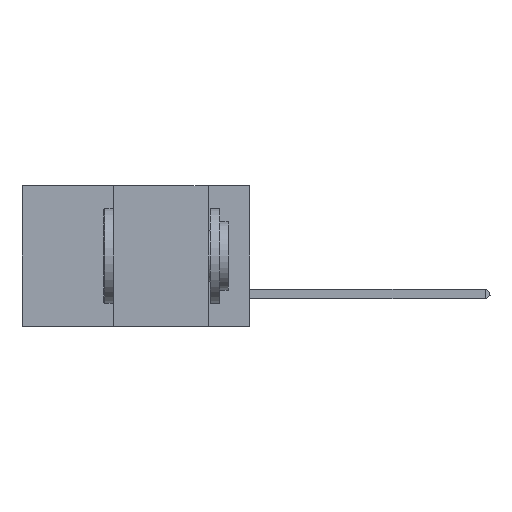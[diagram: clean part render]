
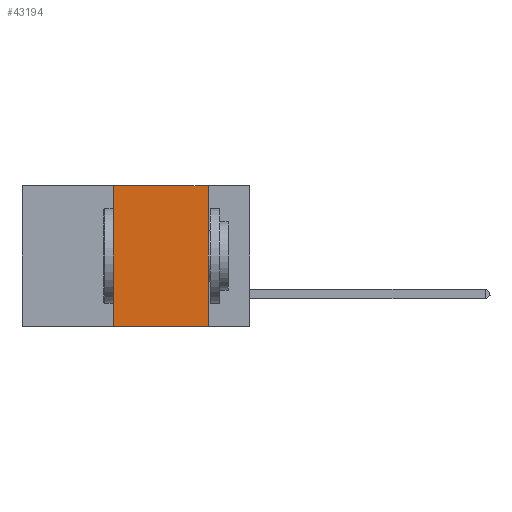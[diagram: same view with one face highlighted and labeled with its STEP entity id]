
A CAD part, left-side view. The second image highlights one B-rep face of the part: STEP entity #43194.
In plain terms, the highlighted planar face has unit normal (-1, 0, 0).
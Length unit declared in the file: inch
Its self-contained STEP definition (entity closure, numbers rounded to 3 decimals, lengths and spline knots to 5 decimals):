
#2362 = ORIENTED_EDGE ( 'NONE', *, *, #32262, .F. ) ;
#2942 = CARTESIAN_POINT ( 'NONE',  ( 0., 0.36, 0. ) ) ;
#3482 = VECTOR ( 'NONE', #45994, 39.37008 ) ;
#4305 = FACE_OUTER_BOUND ( 'NONE', #25678, .T. ) ;
#5193 = VECTOR ( 'NONE', #19960, 39.37008 ) ;
#6873 = VERTEX_POINT ( 'NONE', #46097 ) ;
#8405 = EDGE_CURVE ( 'NONE', #32016, #39889, #25907, .T. ) ;
#8992 = CARTESIAN_POINT ( 'NONE',  ( 0., 0.36, 0. ) ) ;
#10784 = CARTESIAN_POINT ( 'NONE',  ( 0., 0.6, 0. ) ) ;
#12730 = AXIS2_PLACEMENT_3D ( 'NONE', #10784, #32398, #21887 ) ;
#13136 = EDGE_CURVE ( 'NONE', #6873, #39889, #23734, .T. ) ;
#13814 = LINE ( 'NONE', #16260, #5193 ) ;
#16260 = CARTESIAN_POINT ( 'NONE',  ( 0., 0.6, 0. ) ) ;
#19960 = DIRECTION ( 'NONE',  ( 0., -1., 0. ) ) ;
#20381 = DIRECTION ( 'NONE',  ( 0., 0., -1. ) ) ;
#21887 = DIRECTION ( 'NONE',  ( 0., 0., -1. ) ) ;
#22038 = CARTESIAN_POINT ( 'NONE',  ( 0., 0.11, 0. ) ) ;
#23734 = LINE ( 'NONE', #25913, #46881 ) ;
#25525 = EDGE_CURVE ( 'NONE', #27314, #32016, #13814, .T. ) ;
#25602 = DIRECTION ( 'NONE',  ( 0., -1., 0. ) ) ;
#25678 = EDGE_LOOP ( 'NONE', ( #39669, #37157, #2362, #38291 ) ) ;
#25907 = LINE ( 'NONE', #35090, #40384 ) ;
#25913 = CARTESIAN_POINT ( 'NONE',  ( 0., 0.6, -0.37 ) ) ;
#27314 = VERTEX_POINT ( 'NONE', #2942 ) ;
#30850 = CARTESIAN_POINT ( 'NONE',  ( 0., 0.11, -0.37 ) ) ;
#32016 = VERTEX_POINT ( 'NONE', #22038 ) ;
#32262 = EDGE_CURVE ( 'NONE', #6873, #27314, #47351, .T. ) ;
#32398 = DIRECTION ( 'NONE',  ( 1., 0., 0. ) ) ;
#35090 = CARTESIAN_POINT ( 'NONE',  ( 0., 0.11, 0. ) ) ;
#37157 = ORIENTED_EDGE ( 'NONE', *, *, #25525, .F. ) ;
#38291 = ORIENTED_EDGE ( 'NONE', *, *, #13136, .T. ) ;
#39669 = ORIENTED_EDGE ( 'NONE', *, *, #8405, .F. ) ;
#39889 = VERTEX_POINT ( 'NONE', #30850 ) ;
#40384 = VECTOR ( 'NONE', #20381, 39.37008 ) ;
#43194 = ADVANCED_FACE ( 'NONE', ( #4305 ), #44066, .F. ) ;
#44066 = PLANE ( 'NONE',  #12730 ) ;
#45994 = DIRECTION ( 'NONE',  ( 0., 0., 1. ) ) ;
#46097 = CARTESIAN_POINT ( 'NONE',  ( 0., 0.36, -0.37 ) ) ;
#46881 = VECTOR ( 'NONE', #25602, 39.37008 ) ;
#47351 = LINE ( 'NONE', #8992, #3482 ) ;
